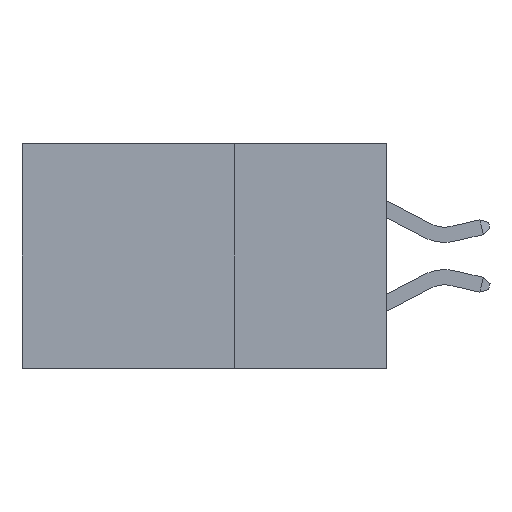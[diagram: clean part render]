
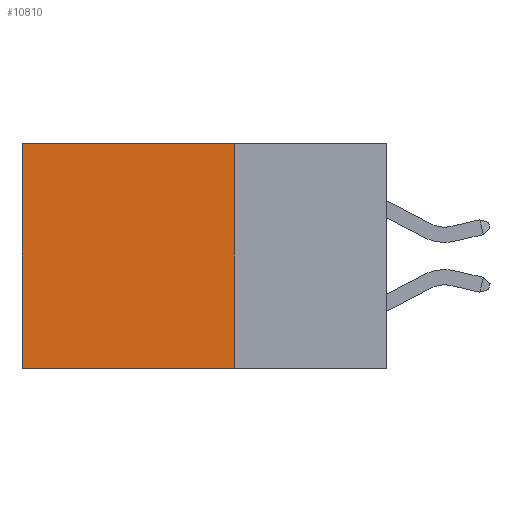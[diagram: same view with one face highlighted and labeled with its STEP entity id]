
A CAD part, left-side view. The second image highlights one B-rep face of the part: STEP entity #10810.
In plain terms, the highlighted planar face has unit normal (-1, 0, 0).
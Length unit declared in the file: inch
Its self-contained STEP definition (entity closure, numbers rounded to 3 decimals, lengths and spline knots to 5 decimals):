
#86 = VECTOR ( 'NONE', #6504, 39.37008 ) ;
#782 = DIRECTION ( 'NONE',  ( 0., 1., 0. ) ) ;
#830 = CARTESIAN_POINT ( 'NONE',  ( 0.298, 0.25, 0. ) ) ;
#1166 = DIRECTION ( 'NONE',  ( 0., 1., 0. ) ) ;
#1189 = LINE ( 'NONE', #830, #4580 ) ;
#1397 = DIRECTION ( 'NONE',  ( 0., 0., -1. ) ) ;
#1612 = CARTESIAN_POINT ( 'NONE',  ( 0.298, 0.25, 0. ) ) ;
#1697 = CARTESIAN_POINT ( 'NONE',  ( 0.298, 0.25, 0. ) ) ;
#2455 = ORIENTED_EDGE ( 'NONE', *, *, #3636, .F. ) ;
#3138 = ORIENTED_EDGE ( 'NONE', *, *, #4844, .T. ) ;
#3283 = ORIENTED_EDGE ( 'NONE', *, *, #9647, .T. ) ;
#3424 = ORIENTED_EDGE ( 'NONE', *, *, #3985, .F. ) ;
#3636 = EDGE_CURVE ( 'NONE', #7705, #4483, #1189, .T. ) ;
#3682 = CARTESIAN_POINT ( 'NONE',  ( 0.298, 0.25, -0.37 ) ) ;
#3905 = CARTESIAN_POINT ( 'NONE',  ( 0.298, 0.6, 0. ) ) ;
#3985 = EDGE_CURVE ( 'NONE', #4483, #4028, #5777, .T. ) ;
#4028 = VERTEX_POINT ( 'NONE', #6385 ) ;
#4483 = VERTEX_POINT ( 'NONE', #9162 ) ;
#4509 = LINE ( 'NONE', #3905, #86 ) ;
#4580 = VECTOR ( 'NONE', #6613, 39.37008 ) ;
#4752 = CARTESIAN_POINT ( 'NONE',  ( 0.298, 0.6, 0. ) ) ;
#4844 = EDGE_CURVE ( 'NONE', #7705, #7074, #8131, .T. ) ;
#5647 = EDGE_LOOP ( 'NONE', ( #3283, #3424, #2455, #3138 ) ) ;
#5777 = LINE ( 'NONE', #3682, #7216 ) ;
#6250 = DIRECTION ( 'NONE',  ( 1., 0., 0. ) ) ;
#6385 = CARTESIAN_POINT ( 'NONE',  ( 0.298, 0.6, -0.37 ) ) ;
#6504 = DIRECTION ( 'NONE',  ( 0., 0., -1. ) ) ;
#6613 = DIRECTION ( 'NONE',  ( 0., 0., -1. ) ) ;
#7074 = VERTEX_POINT ( 'NONE', #4752 ) ;
#7089 = VECTOR ( 'NONE', #782, 39.37008 ) ;
#7216 = VECTOR ( 'NONE', #1166, 39.37008 ) ;
#7705 = VERTEX_POINT ( 'NONE', #1697 ) ;
#7978 = CARTESIAN_POINT ( 'NONE',  ( 0.298, 0.25, 0. ) ) ;
#8131 = LINE ( 'NONE', #1612, #7089 ) ;
#8801 = PLANE ( 'NONE',  #9031 ) ;
#9031 = AXIS2_PLACEMENT_3D ( 'NONE', #7978, #6250, #1397 ) ;
#9162 = CARTESIAN_POINT ( 'NONE',  ( 0.298, 0.25, -0.37 ) ) ;
#9647 = EDGE_CURVE ( 'NONE', #7074, #4028, #4509, .T. ) ;
#9812 = FACE_OUTER_BOUND ( 'NONE', #5647, .T. ) ;
#10810 = ADVANCED_FACE ( 'NONE', ( #9812 ), #8801, .F. ) ;
